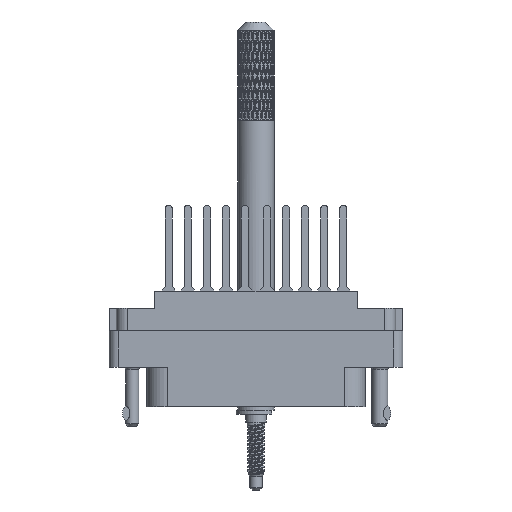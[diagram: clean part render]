
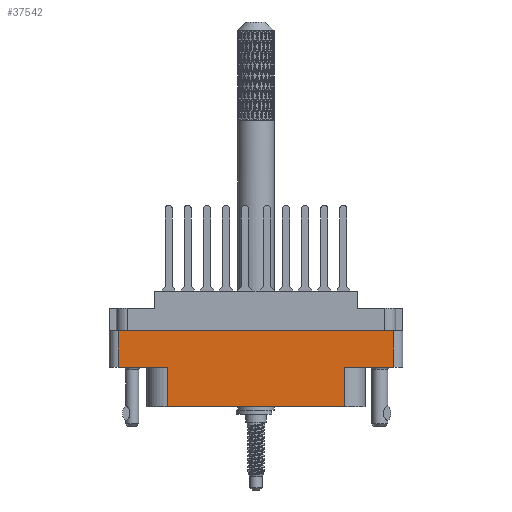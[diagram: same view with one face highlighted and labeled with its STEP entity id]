
A CAD part, front view. The second image highlights one B-rep face of the part: STEP entity #37542.
In plain terms, the highlighted planar face has unit normal (0, -1, 0).
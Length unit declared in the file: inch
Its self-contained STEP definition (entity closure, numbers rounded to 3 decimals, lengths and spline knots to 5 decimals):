
#6198 = CARTESIAN_POINT ( 'NONE',  ( 0.938, -0.438, -0.789 ) ) ;
#6847 = VERTEX_POINT ( 'NONE', #59783 ) ;
#20747 = VERTEX_POINT ( 'NONE', #43205 ) ;
#21120 = CARTESIAN_POINT ( 'NONE',  ( -0.604, -0.438, -0.789 ) ) ;
#23671 = DIRECTION ( 'NONE',  ( 0., 0., 1. ) ) ;
#25512 = CARTESIAN_POINT ( 'NONE',  ( 0.604, -0.438, -0.789 ) ) ;
#26053 = ORIENTED_EDGE ( 'NONE', *, *, #98175, .T. ) ;
#26226 = VERTEX_POINT ( 'NONE', #68900 ) ;
#30873 = CARTESIAN_POINT ( 'NONE',  ( 0., -0.438, -0.52 ) ) ;
#31346 = VECTOR ( 'NONE', #32025, 39.37008 ) ;
#31908 = CARTESIAN_POINT ( 'NONE',  ( 0.604, -0.438, -0.52 ) ) ;
#32025 = DIRECTION ( 'NONE',  ( 1., 0., 0. ) ) ;
#34406 = DIRECTION ( 'NONE',  ( 0., 0., -1. ) ) ;
#36363 = VECTOR ( 'NONE', #39253, 39.37008 ) ;
#37206 = EDGE_LOOP ( 'NONE', ( #106138, #43925, #50679, #26053, #108218, #88454, #64422, #83617 ) ) ;
#37452 = CARTESIAN_POINT ( 'NONE',  ( 0.938, -0.438, -0.52 ) ) ;
#37542 = ADVANCED_FACE ( 'NONE', ( #67505 ), #94201, .T. ) ;
#39253 = DIRECTION ( 'NONE',  ( -1., 0., 0. ) ) ;
#40389 = CARTESIAN_POINT ( 'NONE',  ( 0., -0.438, -0.52 ) ) ;
#42031 = CARTESIAN_POINT ( 'NONE',  ( -1., -0.438, -0.789 ) ) ;
#42660 = CARTESIAN_POINT ( 'NONE',  ( -1., -0.438, -0.789 ) ) ;
#43047 = DIRECTION ( 'NONE',  ( 1., 0., 0. ) ) ;
#43205 = CARTESIAN_POINT ( 'NONE',  ( -0.938, -0.438, -0.52 ) ) ;
#43554 = EDGE_CURVE ( 'NONE', #26226, #6847, #89911, .T. ) ;
#43603 = VECTOR ( 'NONE', #48344, 39.37008 ) ;
#43925 = ORIENTED_EDGE ( 'NONE', *, *, #86251, .T. ) ;
#46567 = EDGE_CURVE ( 'NONE', #58667, #79573, #49967, .T. ) ;
#47883 = EDGE_CURVE ( 'NONE', #57996, #79573, #83573, .T. ) ;
#48344 = DIRECTION ( 'NONE',  ( 1., 0., 0. ) ) ;
#48726 = CARTESIAN_POINT ( 'NONE',  ( 0., -0.438, -0.268 ) ) ;
#49967 = LINE ( 'NONE', #30873, #36363 ) ;
#49980 = VECTOR ( 'NONE', #23671, 39.37008 ) ;
#50679 = ORIENTED_EDGE ( 'NONE', *, *, #106234, .T. ) ;
#51816 = VECTOR ( 'NONE', #34406, 39.37008 ) ;
#55859 = EDGE_CURVE ( 'NONE', #58667, #6847, #111207, .T. ) ;
#57096 = EDGE_CURVE ( 'NONE', #98127, #57996, #71562, .T. ) ;
#57277 = LINE ( 'NONE', #40389, #31346 ) ;
#57996 = VERTEX_POINT ( 'NONE', #25512 ) ;
#58667 = VERTEX_POINT ( 'NONE', #37452 ) ;
#59783 = CARTESIAN_POINT ( 'NONE',  ( 0.938, -0.438, -0.268 ) ) ;
#59956 = VECTOR ( 'NONE', #64812, 39.37008 ) ;
#59982 = CARTESIAN_POINT ( 'NONE',  ( -0.938, -0.438, -0.789 ) ) ;
#64422 = ORIENTED_EDGE ( 'NONE', *, *, #46567, .F. ) ;
#64812 = DIRECTION ( 'NONE',  ( 0., 0., -1. ) ) ;
#65907 = CARTESIAN_POINT ( 'NONE',  ( -0.604, -0.438, -0.52 ) ) ;
#67505 = FACE_OUTER_BOUND ( 'NONE', #37206, .T. ) ;
#68900 = CARTESIAN_POINT ( 'NONE',  ( -0.938, -0.438, -0.268 ) ) ;
#71562 = LINE ( 'NONE', #42660, #90583 ) ;
#74957 = LINE ( 'NONE', #59982, #51816 ) ;
#79573 = VERTEX_POINT ( 'NONE', #31908 ) ;
#80406 = VERTEX_POINT ( 'NONE', #65907 ) ;
#83573 = LINE ( 'NONE', #87149, #94481 ) ;
#83617 = ORIENTED_EDGE ( 'NONE', *, *, #55859, .T. ) ;
#85809 = LINE ( 'NONE', #90738, #59956 ) ;
#86251 = EDGE_CURVE ( 'NONE', #26226, #20747, #74957, .T. ) ;
#87149 = CARTESIAN_POINT ( 'NONE',  ( 0.604, -0.438, -0.52 ) ) ;
#87518 = DIRECTION ( 'NONE',  ( 0., 0., 1. ) ) ;
#88454 = ORIENTED_EDGE ( 'NONE', *, *, #47883, .T. ) ;
#88548 = AXIS2_PLACEMENT_3D ( 'NONE', #42031, #102928, #111684 ) ;
#89911 = LINE ( 'NONE', #48726, #43603 ) ;
#90583 = VECTOR ( 'NONE', #43047, 39.37008 ) ;
#90738 = CARTESIAN_POINT ( 'NONE',  ( -0.604, -0.438, -0.789 ) ) ;
#94201 = PLANE ( 'NONE',  #88548 ) ;
#94481 = VECTOR ( 'NONE', #87518, 39.37008 ) ;
#98127 = VERTEX_POINT ( 'NONE', #21120 ) ;
#98175 = EDGE_CURVE ( 'NONE', #80406, #98127, #85809, .T. ) ;
#102928 = DIRECTION ( 'NONE',  ( 0., -1., 0. ) ) ;
#106138 = ORIENTED_EDGE ( 'NONE', *, *, #43554, .F. ) ;
#106234 = EDGE_CURVE ( 'NONE', #20747, #80406, #57277, .T. ) ;
#108218 = ORIENTED_EDGE ( 'NONE', *, *, #57096, .T. ) ;
#111207 = LINE ( 'NONE', #6198, #49980 ) ;
#111684 = DIRECTION ( 'NONE',  ( 0., 0., -1. ) ) ;
